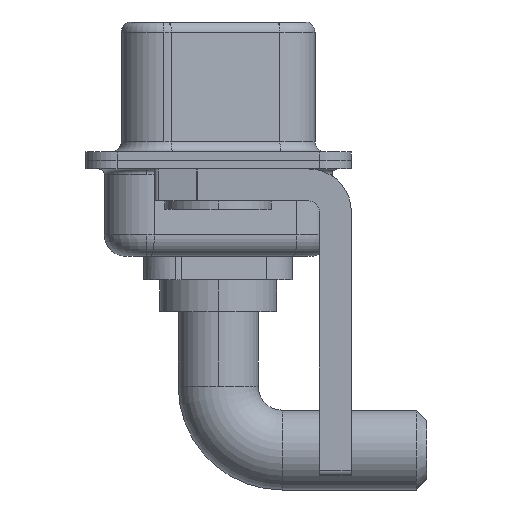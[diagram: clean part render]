
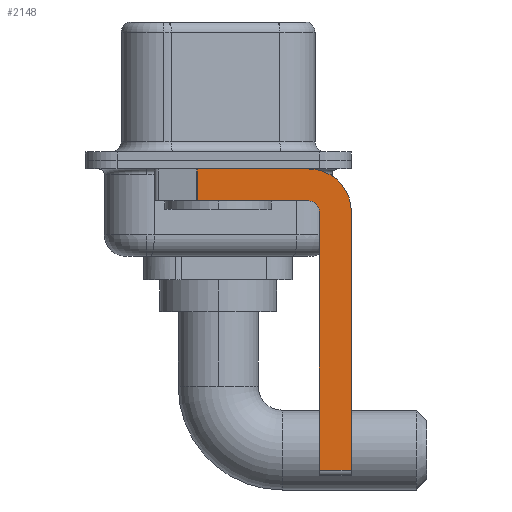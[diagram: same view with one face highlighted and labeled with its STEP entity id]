
A CAD part, left-side view. The second image highlights one B-rep face of the part: STEP entity #2148.
In plain terms, the highlighted planar face has unit normal (-1, 0, 0).
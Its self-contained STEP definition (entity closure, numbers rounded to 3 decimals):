
#312 = DIRECTION ( 'NONE',  ( 0., -1., 0. ) ) ;
#344 = DIRECTION ( 'NONE',  ( 0., 0., 1. ) ) ;
#593 = DIRECTION ( 'NONE',  ( 0., 0., -1. ) ) ;
#827 = PLANE ( 'NONE',  #9469 ) ;
#1242 = VERTEX_POINT ( 'NONE', #2610 ) ;
#1295 = VECTOR ( 'NONE', #312, 1000. ) ;
#1435 = ORIENTED_EDGE ( 'NONE', *, *, #2078, .F. ) ;
#1474 = AXIS2_PLACEMENT_3D ( 'NONE', #8670, #15316, #15235 ) ;
#1565 = CARTESIAN_POINT ( 'NONE',  ( -2.9, 0.978, -1.9 ) ) ;
#1864 = LINE ( 'NONE', #7075, #5156 ) ;
#2078 = EDGE_CURVE ( 'NONE', #16311, #10073, #11365, .T. ) ;
#2103 = VERTEX_POINT ( 'NONE', #11981 ) ;
#2116 = EDGE_CURVE ( 'NONE', #2103, #3133, #14476, .T. ) ;
#2148 = ADVANCED_FACE ( 'NONE', ( #7316 ), #827, .F. ) ;
#2257 = CARTESIAN_POINT ( 'NONE',  ( -2.9, -4.25, -2.4 ) ) ;
#2381 = CARTESIAN_POINT ( 'NONE',  ( -2.9, -6.25, -2.4 ) ) ;
#2610 = CARTESIAN_POINT ( 'NONE',  ( -2.9, -4.75, -2.4 ) ) ;
#2732 = VERTEX_POINT ( 'NONE', #7212 ) ;
#2740 = LINE ( 'NONE', #3074, #13853 ) ;
#2789 = CARTESIAN_POINT ( 'NONE',  ( -2.9, -4.25, -14.55 ) ) ;
#2838 = CIRCLE ( 'NONE', #1474, 0.5 ) ;
#3074 = CARTESIAN_POINT ( 'NONE',  ( -2.9, -4.75, -14.8 ) ) ;
#3133 = VERTEX_POINT ( 'NONE', #14048 ) ;
#3268 = CARTESIAN_POINT ( 'NONE',  ( -2.9, -4.25, -0.4 ) ) ;
#3314 = DIRECTION ( 'NONE',  ( 0., -1., 0. ) ) ;
#3551 = VECTOR ( 'NONE', #5631, 1000. ) ;
#3648 = CARTESIAN_POINT ( 'NONE',  ( -2.9, -4.25, -1.9 ) ) ;
#4265 = LINE ( 'NONE', #14668, #5829 ) ;
#4486 = ORIENTED_EDGE ( 'NONE', *, *, #12973, .F. ) ;
#4886 = CARTESIAN_POINT ( 'NONE',  ( -2.9, -6.25, -2.4 ) ) ;
#5156 = VECTOR ( 'NONE', #3314, 1000. ) ;
#5424 = ORIENTED_EDGE ( 'NONE', *, *, #7005, .F. ) ;
#5631 = DIRECTION ( 'NONE',  ( 0., 1., 0. ) ) ;
#5829 = VECTOR ( 'NONE', #593, 1000. ) ;
#6036 = DIRECTION ( 'NONE',  ( 1., 0., 0. ) ) ;
#6434 = EDGE_CURVE ( 'NONE', #2732, #14433, #4265, .T. ) ;
#6605 = ORIENTED_EDGE ( 'NONE', *, *, #13613, .F. ) ;
#6811 = CARTESIAN_POINT ( 'NONE',  ( -2.9, -4.25, -2.4 ) ) ;
#7005 = EDGE_CURVE ( 'NONE', #1242, #11880, #2838, .T. ) ;
#7075 = CARTESIAN_POINT ( 'NONE',  ( -2.9, 3., -0.4 ) ) ;
#7212 = CARTESIAN_POINT ( 'NONE',  ( -2.9, 0.978, -0.4 ) ) ;
#7316 = FACE_OUTER_BOUND ( 'NONE', #10427, .T. ) ;
#7560 = EDGE_CURVE ( 'NONE', #10073, #3133, #13057, .T. ) ;
#7860 = ORIENTED_EDGE ( 'NONE', *, *, #16551, .F. ) ;
#8174 = ORIENTED_EDGE ( 'NONE', *, *, #7560, .F. ) ;
#8655 = AXIS2_PLACEMENT_3D ( 'NONE', #6811, #13526, #9438 ) ;
#8670 = CARTESIAN_POINT ( 'NONE',  ( -2.9, -4.25, -2.4 ) ) ;
#9438 = DIRECTION ( 'NONE',  ( 0., 0., -1. ) ) ;
#9469 = AXIS2_PLACEMENT_3D ( 'NONE', #2257, #6036, #14910 ) ;
#10073 = VERTEX_POINT ( 'NONE', #2381 ) ;
#10338 = ORIENTED_EDGE ( 'NONE', *, *, #6434, .T. ) ;
#10427 = EDGE_LOOP ( 'NONE', ( #6605, #10338, #7860, #5424, #4486, #16287, #8174, #1435 ) ) ;
#11365 = CIRCLE ( 'NONE', #8655, 2. ) ;
#11440 = DIRECTION ( 'NONE',  ( 0., 0., -1. ) ) ;
#11679 = LINE ( 'NONE', #13449, #3551 ) ;
#11880 = VERTEX_POINT ( 'NONE', #3648 ) ;
#11981 = CARTESIAN_POINT ( 'NONE',  ( -2.9, -4.75, -14.55 ) ) ;
#12973 = EDGE_CURVE ( 'NONE', #2103, #1242, #2740, .T. ) ;
#13057 = LINE ( 'NONE', #4886, #14846 ) ;
#13449 = CARTESIAN_POINT ( 'NONE',  ( -2.9, -4.25, -1.9 ) ) ;
#13526 = DIRECTION ( 'NONE',  ( 1., 0., 0. ) ) ;
#13613 = EDGE_CURVE ( 'NONE', #2732, #16311, #1864, .T. ) ;
#13853 = VECTOR ( 'NONE', #344, 1000. ) ;
#14048 = CARTESIAN_POINT ( 'NONE',  ( -2.9, -6.25, -14.55 ) ) ;
#14433 = VERTEX_POINT ( 'NONE', #1565 ) ;
#14476 = LINE ( 'NONE', #2789, #1295 ) ;
#14668 = CARTESIAN_POINT ( 'NONE',  ( -2.9, 0.978, -1.9 ) ) ;
#14846 = VECTOR ( 'NONE', #11440, 1000. ) ;
#14910 = DIRECTION ( 'NONE',  ( 0., 0., -1. ) ) ;
#15235 = DIRECTION ( 'NONE',  ( 0., 0., 1. ) ) ;
#15316 = DIRECTION ( 'NONE',  ( -1., 0., 0. ) ) ;
#16287 = ORIENTED_EDGE ( 'NONE', *, *, #2116, .T. ) ;
#16311 = VERTEX_POINT ( 'NONE', #3268 ) ;
#16551 = EDGE_CURVE ( 'NONE', #11880, #14433, #11679, .T. ) ;
